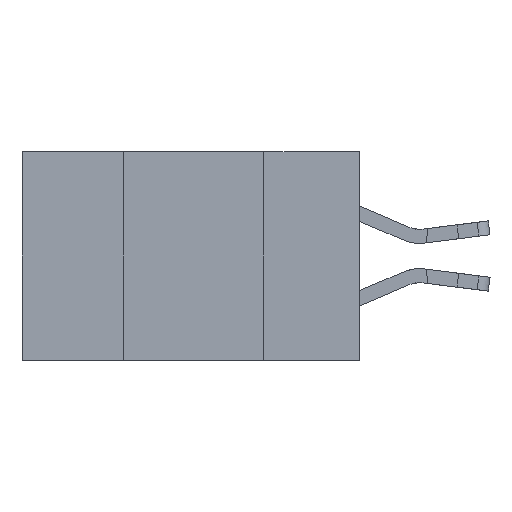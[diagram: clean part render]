
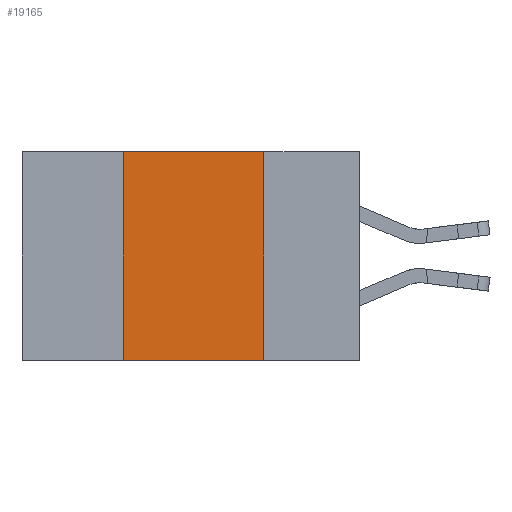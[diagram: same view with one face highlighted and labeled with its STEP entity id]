
A CAD part, left-side view. The second image highlights one B-rep face of the part: STEP entity #19165.
In plain terms, the highlighted planar face has unit normal (-1, 0, 0).
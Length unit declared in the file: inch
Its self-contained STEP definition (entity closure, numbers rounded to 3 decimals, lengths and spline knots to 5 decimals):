
#2200 = EDGE_CURVE ( 'NONE', #19113, #21247, #11165, .T. ) ;
#3144 = VECTOR ( 'NONE', #19931, 39.37008 ) ;
#3176 = CARTESIAN_POINT ( 'NONE',  ( 0., 0.17, 0. ) ) ;
#3891 = PLANE ( 'NONE',  #26435 ) ;
#5820 = EDGE_CURVE ( 'NONE', #14632, #19113, #7330, .T. ) ;
#7330 = LINE ( 'NONE', #22022, #20277 ) ;
#9716 = CARTESIAN_POINT ( 'NONE',  ( 0., 0.42, 0. ) ) ;
#9777 = CARTESIAN_POINT ( 'NONE',  ( 0., 0.17, -0.37 ) ) ;
#9974 = FACE_OUTER_BOUND ( 'NONE', #16159, .T. ) ;
#11165 = LINE ( 'NONE', #25621, #16491 ) ;
#11177 = CARTESIAN_POINT ( 'NONE',  ( 0., 0.42, -0.37 ) ) ;
#11251 = EDGE_CURVE ( 'NONE', #14632, #11455, #22039, .T. ) ;
#11300 = DIRECTION ( 'NONE',  ( 0., -1., 0. ) ) ;
#11455 = VERTEX_POINT ( 'NONE', #9777 ) ;
#11597 = LINE ( 'NONE', #13876, #3144 ) ;
#12210 = ORIENTED_EDGE ( 'NONE', *, *, #2200, .F. ) ;
#13240 = ORIENTED_EDGE ( 'NONE', *, *, #5820, .F. ) ;
#13564 = ORIENTED_EDGE ( 'NONE', *, *, #19089, .F. ) ;
#13876 = CARTESIAN_POINT ( 'NONE',  ( 0., 0.17, 0. ) ) ;
#14632 = VERTEX_POINT ( 'NONE', #11177 ) ;
#15521 = DIRECTION ( 'NONE',  ( 0., 0., 1. ) ) ;
#16159 = EDGE_LOOP ( 'NONE', ( #13564, #12210, #13240, #22262 ) ) ;
#16491 = VECTOR ( 'NONE', #11300, 39.37008 ) ;
#16929 = VECTOR ( 'NONE', #23815, 39.37008 ) ;
#18686 = DIRECTION ( 'NONE',  ( 1., 0., 0. ) ) ;
#19089 = EDGE_CURVE ( 'NONE', #21247, #11455, #11597, .T. ) ;
#19113 = VERTEX_POINT ( 'NONE', #9716 ) ;
#19165 = ADVANCED_FACE ( 'NONE', ( #9974 ), #3891, .F. ) ;
#19931 = DIRECTION ( 'NONE',  ( 0., 0., -1. ) ) ;
#20277 = VECTOR ( 'NONE', #15521, 39.37008 ) ;
#21247 = VERTEX_POINT ( 'NONE', #3176 ) ;
#22022 = CARTESIAN_POINT ( 'NONE',  ( 0., 0.42, 0. ) ) ;
#22039 = LINE ( 'NONE', #23959, #16929 ) ;
#22262 = ORIENTED_EDGE ( 'NONE', *, *, #11251, .T. ) ;
#22642 = CARTESIAN_POINT ( 'NONE',  ( 0., 0.6, 0. ) ) ;
#23815 = DIRECTION ( 'NONE',  ( 0., -1., 0. ) ) ;
#23959 = CARTESIAN_POINT ( 'NONE',  ( 0., 0.6, -0.37 ) ) ;
#25621 = CARTESIAN_POINT ( 'NONE',  ( 0., 0.6, 0. ) ) ;
#26435 = AXIS2_PLACEMENT_3D ( 'NONE', #22642, #18686, #26457 ) ;
#26457 = DIRECTION ( 'NONE',  ( 0., 0., -1. ) ) ;
